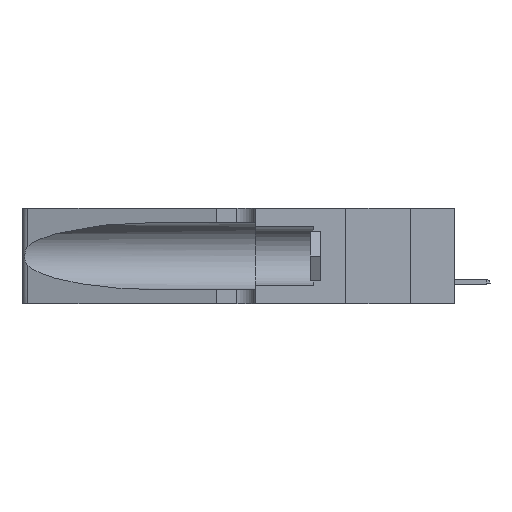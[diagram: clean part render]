
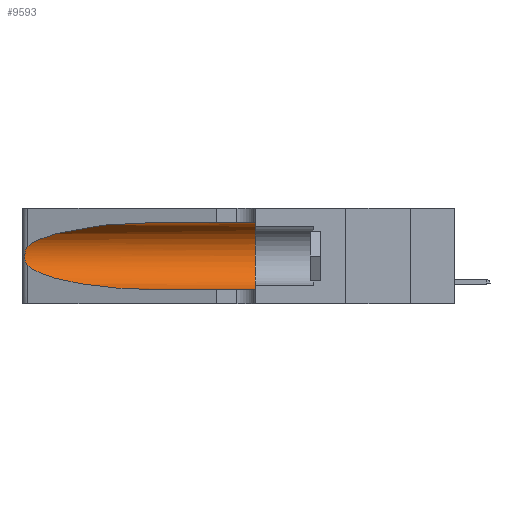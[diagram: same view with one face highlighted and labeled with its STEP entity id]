
A CAD part, left-side view. The second image highlights one B-rep face of the part: STEP entity #9593.
In plain terms, the highlighted cylindrical face has radius 3.308 mm (diameter 6.617 mm), a partial arc.
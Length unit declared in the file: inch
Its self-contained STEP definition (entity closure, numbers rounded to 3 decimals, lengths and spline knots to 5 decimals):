
#2126 = CARTESIAN_POINT ( 'NONE',  ( 0.25856, 1.23593, 0.16098 ) ) ;
#2454 = ORIENTED_EDGE ( 'NONE', *, *, #18762, .T. ) ;
#2474 = VERTEX_POINT ( 'NONE', #27366 ) ;
#2529 = VERTEX_POINT ( 'NONE', #3375 ) ;
#3375 = CARTESIAN_POINT ( 'NONE',  ( 0.1305, 0.72297, 0.05475 ) ) ;
#3462 = CARTESIAN_POINT ( 'NONE',  ( 0.18966, 0.96281, 0.05475 ) ) ;
#3561 = EDGE_CURVE ( 'NONE', #6032, #20991, #18696, .T. ) ;
#3614 = CARTESIAN_POINT ( 'NONE',  ( 0.25487, 1.22718, 0.14631 ) ) ;
#3981 = DIRECTION ( 'NONE',  ( 0., 0., 1. ) ) ;
#3989 = AXIS2_PLACEMENT_3D ( 'NONE', #21387, #19228, #3981 ) ;
#4024 = CARTESIAN_POINT ( 'NONE',  ( 0.26075, 1.23896, 0.178 ) ) ;
#4299 = CARTESIAN_POINT ( 'NONE',  ( 0.25787, 1.23484, 0.2124 ) ) ;
#4364 = CARTESIAN_POINT ( 'NONE',  ( 0.18966, 0.96281, 0.31525 ) ) ;
#4444 = CARTESIAN_POINT ( 'NONE',  ( 0.25555, 1.22994, 0.2215 ) ) ;
#5142 = DIRECTION ( 'NONE',  ( 0., -1., 0. ) ) ;
#5456 = LINE ( 'NONE', #9614, #21851 ) ;
#5468 = VERTEX_POINT ( 'NONE', #19524 ) ;
#5978 =( BOUNDED_CURVE ( )  B_SPLINE_CURVE ( 3, ( #27941, #4364, #8388, #8671 ),
 .UNSPECIFIED., .F., .F. ) 
 B_SPLINE_CURVE_WITH_KNOTS ( ( 4, 4 ),
 ( 1.5708, 2.84003 ),
 .UNSPECIFIED. ) 
 CURVE ( )  GEOMETRIC_REPRESENTATION_ITEM ( )  RATIONAL_B_SPLINE_CURVE ( ( 1., 0.87, 0.87, 1. ) ) 
 REPRESENTATION_ITEM ( '' )  );
#6032 = VERTEX_POINT ( 'NONE', #22916 ) ;
#6049 = CARTESIAN_POINT ( 'NONE',  ( 0.25487, 1.22718, 0.22369 ) ) ;
#7295 = CARTESIAN_POINT ( 'NONE',  ( 0.1305, 1.61858, 0.05475 ) ) ;
#8388 = CARTESIAN_POINT ( 'NONE',  ( 0.2373, 1.15595, 0.28018 ) ) ;
#8460 = CARTESIAN_POINT ( 'NONE',  ( 0.25639, 1.23186, 0.15144 ) ) ;
#8671 = CARTESIAN_POINT ( 'NONE',  ( 0.25487, 1.22718, 0.22369 ) ) ;
#9451 = LINE ( 'NONE', #7295, #15228 ) ;
#9593 = ADVANCED_FACE ( 'NONE', ( #12192 ), #22688, .F. ) ;
#9614 = CARTESIAN_POINT ( 'NONE',  ( 0.1305, 1.61858, 0.31525 ) ) ;
#9927 = CARTESIAN_POINT ( 'NONE',  ( 0.1305, 0.72297, 0.05475 ) ) ;
#10492 = EDGE_CURVE ( 'NONE', #5468, #11290, #25464, .T. ) ;
#10630 = CARTESIAN_POINT ( 'NONE',  ( 0.26017, 1.23833, 0.17102 ) ) ;
#10868 = EDGE_CURVE ( 'NONE', #2474, #6032, #5456, .T. ) ;
#11047 = CARTESIAN_POINT ( 'NONE',  ( 0.25555, 1.22993, 0.14849 ) ) ;
#11290 = VERTEX_POINT ( 'NONE', #23787 ) ;
#11723 = ORIENTED_EDGE ( 'NONE', *, *, #3561, .F. ) ;
#12192 = FACE_OUTER_BOUND ( 'NONE', #13212, .T. ) ;
#13212 = EDGE_LOOP ( 'NONE', ( #19080, #21785, #23876, #2454, #11723, #18566 ) ) ;
#15228 = VECTOR ( 'NONE', #5142, 39.37008 ) ;
#16080 = CARTESIAN_POINT ( 'NONE',  ( 0.1305, 0.35, 0.05475 ) ) ;
#16501 = DIRECTION ( 'NONE',  ( 0., -1., 0. ) ) ;
#17237 = CARTESIAN_POINT ( 'NONE',  ( 0.25789, 1.23486, 0.15765 ) ) ;
#17381 = CARTESIAN_POINT ( 'NONE',  ( 0.26075, 1.23896, 0.19203 ) ) ;
#17517 = CARTESIAN_POINT ( 'NONE',  ( 0.25487, 1.22718, 0.14631 ) ) ;
#18566 = ORIENTED_EDGE ( 'NONE', *, *, #10868, .F. ) ;
#18696 = CIRCLE ( 'NONE', #3989, 0.13025 ) ;
#18762 = EDGE_CURVE ( 'NONE', #2529, #20991, #9451, .T. ) ;
#19080 = ORIENTED_EDGE ( 'NONE', *, *, #26112, .T. ) ;
#19228 = DIRECTION ( 'NONE',  ( 0., 1., 0. ) ) ;
#19524 = CARTESIAN_POINT ( 'NONE',  ( 0.25487, 1.22718, 0.22369 ) ) ;
#20590 = CARTESIAN_POINT ( 'NONE',  ( 0.2373, 1.15595, 0.08982 ) ) ;
#20682 = CARTESIAN_POINT ( 'NONE',  ( 0.1305, 1.61858, 0.185 ) ) ;
#20991 = VERTEX_POINT ( 'NONE', #16080 ) ;
#21387 = CARTESIAN_POINT ( 'NONE',  ( 0.1305, 0.35, 0.185 ) ) ;
#21785 = ORIENTED_EDGE ( 'NONE', *, *, #10492, .T. ) ;
#21851 = VECTOR ( 'NONE', #27845, 39.37008 ) ;
#22688 = CYLINDRICAL_SURFACE ( 'NONE', #24539, 0.13025 ) ;
#22916 = CARTESIAN_POINT ( 'NONE',  ( 0.1305, 0.35, 0.31525 ) ) ;
#23787 = CARTESIAN_POINT ( 'NONE',  ( 0.25487, 1.22718, 0.14631 ) ) ;
#23876 = ORIENTED_EDGE ( 'NONE', *, *, #28004, .T. ) ;
#24539 = AXIS2_PLACEMENT_3D ( 'NONE', #20682, #16501, #25263 ) ;
#25263 = DIRECTION ( 'NONE',  ( 0., 0., -1. ) ) ;
#25464 = B_SPLINE_CURVE_WITH_KNOTS ( 'NONE', 3,
 ( #6049, #4444, #25713, #4299, #28151, #28290, #17381, #4024, #10630, #2126, #17237, #8460, #11047, #17517 ),
 .UNSPECIFIED., .F., .F.,
 ( 4, 2, 2, 2, 2, 2, 4 ),
 ( 0., 0.00027, 0.00053, 0.00107, 0.0016, 0.00187, 0.00214 ),
 .UNSPECIFIED. ) ;
#25713 = CARTESIAN_POINT ( 'NONE',  ( 0.25639, 1.23184, 0.21858 ) ) ;
#26112 = EDGE_CURVE ( 'NONE', #2474, #5468, #5978, .T. ) ;
#27366 = CARTESIAN_POINT ( 'NONE',  ( 0.1305, 0.72297, 0.31525 ) ) ;
#27845 = DIRECTION ( 'NONE',  ( 0., -1., 0. ) ) ;
#27941 = CARTESIAN_POINT ( 'NONE',  ( 0.1305, 0.72297, 0.31525 ) ) ;
#28004 = EDGE_CURVE ( 'NONE', #11290, #2529, #28136, .T. ) ;
#28136 =( BOUNDED_CURVE ( )  B_SPLINE_CURVE ( 3, ( #3614, #20590, #3462, #9927 ),
 .UNSPECIFIED., .F., .T. ) 
 B_SPLINE_CURVE_WITH_KNOTS ( ( 4, 4 ),
 ( 3.44316, 4.71239 ),
 .UNSPECIFIED. ) 
 CURVE ( )  GEOMETRIC_REPRESENTATION_ITEM ( )  RATIONAL_B_SPLINE_CURVE ( ( 1., 0.87, 0.87, 1. ) ) 
 REPRESENTATION_ITEM ( '' )  );
#28151 = CARTESIAN_POINT ( 'NONE',  ( 0.25854, 1.2359, 0.20912 ) ) ;
#28290 = CARTESIAN_POINT ( 'NONE',  ( 0.26018, 1.23835, 0.19895 ) ) ;
